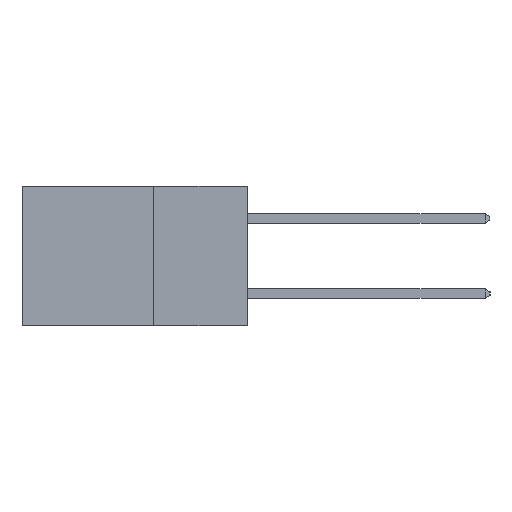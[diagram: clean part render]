
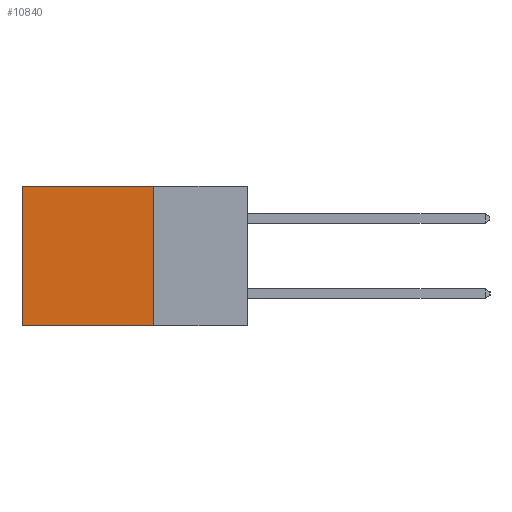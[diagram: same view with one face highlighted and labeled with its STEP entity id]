
A CAD part, left-side view. The second image highlights one B-rep face of the part: STEP entity #10840.
In plain terms, the highlighted planar face has unit normal (-1, 0, 0).
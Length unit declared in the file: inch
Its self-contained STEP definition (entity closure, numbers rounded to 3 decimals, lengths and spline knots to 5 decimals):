
#952 = EDGE_CURVE ( 'NONE', #14957, #13800, #15784, .T. ) ;
#1248 = ORIENTED_EDGE ( 'NONE', *, *, #12894, .F. ) ;
#2710 = AXIS2_PLACEMENT_3D ( 'NONE', #12418, #7811, #18722 ) ;
#4837 = EDGE_CURVE ( 'NONE', #17462, #14957, #9826, .T. ) ;
#5591 = VECTOR ( 'NONE', #8514, 39.37008 ) ;
#5753 = ORIENTED_EDGE ( 'NONE', *, *, #952, .T. ) ;
#6030 = CARTESIAN_POINT ( 'NONE',  ( 0.2615, 0.25, -0.37 ) ) ;
#6629 = EDGE_LOOP ( 'NONE', ( #5753, #11253, #1248, #9729 ) ) ;
#6689 = FACE_OUTER_BOUND ( 'NONE', #6629, .T. ) ;
#7094 = VECTOR ( 'NONE', #10386, 39.37008 ) ;
#7338 = CARTESIAN_POINT ( 'NONE',  ( 0.2615, 0.6, 0. ) ) ;
#7811 = DIRECTION ( 'NONE',  ( 1., 0., 0. ) ) ;
#7836 = VECTOR ( 'NONE', #12406, 39.37008 ) ;
#8514 = DIRECTION ( 'NONE',  ( 0., 1., 0. ) ) ;
#9380 = DIRECTION ( 'NONE',  ( 0., 0., -1. ) ) ;
#9609 = VERTEX_POINT ( 'NONE', #6030 ) ;
#9729 = ORIENTED_EDGE ( 'NONE', *, *, #4837, .T. ) ;
#9826 = LINE ( 'NONE', #13103, #5591 ) ;
#10386 = DIRECTION ( 'NONE',  ( 0., 0., -1. ) ) ;
#10840 = ADVANCED_FACE ( 'NONE', ( #6689 ), #10859, .F. ) ;
#10847 = CARTESIAN_POINT ( 'NONE',  ( 0.2615, 0.25, -0.37 ) ) ;
#10859 = PLANE ( 'NONE',  #2710 ) ;
#11253 = ORIENTED_EDGE ( 'NONE', *, *, #13126, .F. ) ;
#11727 = LINE ( 'NONE', #18156, #7094 ) ;
#11952 = LINE ( 'NONE', #10847, #7836 ) ;
#12406 = DIRECTION ( 'NONE',  ( 0., 1., 0. ) ) ;
#12418 = CARTESIAN_POINT ( 'NONE',  ( 0.2615, 0.25, -0.37 ) ) ;
#12894 = EDGE_CURVE ( 'NONE', #17462, #9609, #11727, .T. ) ;
#13103 = CARTESIAN_POINT ( 'NONE',  ( 0.2615, 0.25, 0. ) ) ;
#13126 = EDGE_CURVE ( 'NONE', #9609, #13800, #11952, .T. ) ;
#13800 = VERTEX_POINT ( 'NONE', #18624 ) ;
#14957 = VERTEX_POINT ( 'NONE', #7338 ) ;
#15276 = VECTOR ( 'NONE', #9380, 39.37008 ) ;
#15784 = LINE ( 'NONE', #18149, #15276 ) ;
#15872 = CARTESIAN_POINT ( 'NONE',  ( 0.2615, 0.25, 0. ) ) ;
#17462 = VERTEX_POINT ( 'NONE', #15872 ) ;
#18149 = CARTESIAN_POINT ( 'NONE',  ( 0.2615, 0.6, -0.37 ) ) ;
#18156 = CARTESIAN_POINT ( 'NONE',  ( 0.2615, 0.25, -0.37 ) ) ;
#18624 = CARTESIAN_POINT ( 'NONE',  ( 0.2615, 0.6, -0.37 ) ) ;
#18722 = DIRECTION ( 'NONE',  ( 0., 0., -1. ) ) ;
